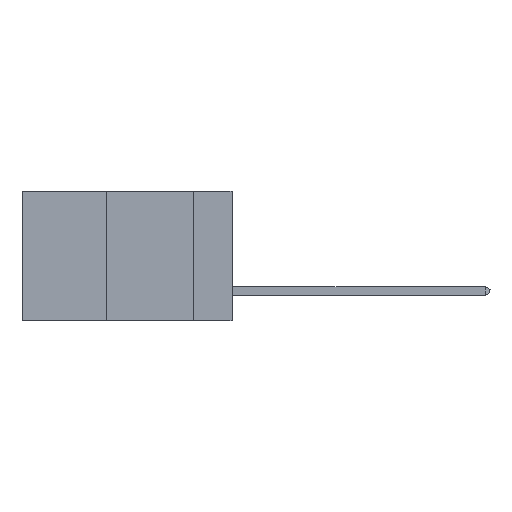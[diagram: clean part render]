
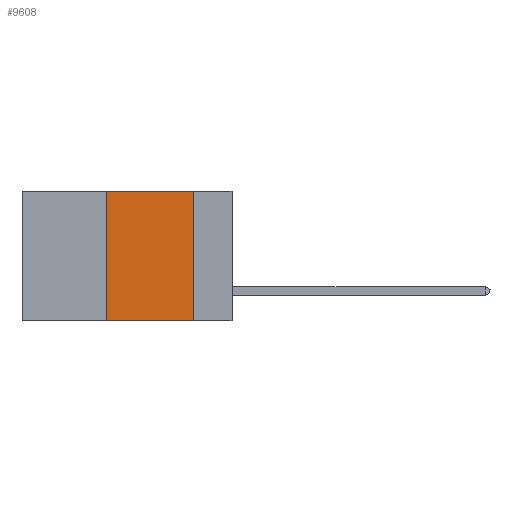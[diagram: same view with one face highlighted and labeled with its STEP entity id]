
A CAD part, left-side view. The second image highlights one B-rep face of the part: STEP entity #9608.
In plain terms, the highlighted planar face has unit normal (-1, 0, 0).
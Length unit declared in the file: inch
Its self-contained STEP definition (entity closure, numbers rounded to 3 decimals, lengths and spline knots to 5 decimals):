
#503 = DIRECTION ( 'NONE',  ( 0., -1., 0. ) ) ;
#2063 = CARTESIAN_POINT ( 'NONE',  ( 0., 0.11, 0. ) ) ;
#2697 = CARTESIAN_POINT ( 'NONE',  ( 0., 0.36, 0. ) ) ;
#3089 = EDGE_CURVE ( 'NONE', #4836, #41034, #37772, .T. ) ;
#3091 = DIRECTION ( 'NONE',  ( 0., -1., 0. ) ) ;
#3403 = CARTESIAN_POINT ( 'NONE',  ( 0., 0.6, 0. ) ) ;
#4161 = CARTESIAN_POINT ( 'NONE',  ( 0., 0.6, -0.37 ) ) ;
#4836 = VERTEX_POINT ( 'NONE', #2063 ) ;
#5991 = LINE ( 'NONE', #4161, #6514 ) ;
#6039 = CARTESIAN_POINT ( 'NONE',  ( 0., 0.6, 0. ) ) ;
#6367 = VECTOR ( 'NONE', #20189, 39.37008 ) ;
#6514 = VECTOR ( 'NONE', #503, 39.37008 ) ;
#7073 = EDGE_CURVE ( 'NONE', #39208, #4836, #10247, .T. ) ;
#7361 = ORIENTED_EDGE ( 'NONE', *, *, #29477, .T. ) ;
#8888 = VECTOR ( 'NONE', #37668, 39.37008 ) ;
#9069 = DIRECTION ( 'NONE',  ( 0., 0., -1. ) ) ;
#9608 = ADVANCED_FACE ( 'NONE', ( #11152 ), #29910, .F. ) ;
#10247 = LINE ( 'NONE', #3403, #39128 ) ;
#10647 = AXIS2_PLACEMENT_3D ( 'NONE', #6039, #33716, #9069 ) ;
#10871 = EDGE_CURVE ( 'NONE', #35455, #39208, #38512, .T. ) ;
#11152 = FACE_OUTER_BOUND ( 'NONE', #34648, .T. ) ;
#12516 = ORIENTED_EDGE ( 'NONE', *, *, #7073, .F. ) ;
#15843 = ORIENTED_EDGE ( 'NONE', *, *, #3089, .F. ) ;
#17462 = ORIENTED_EDGE ( 'NONE', *, *, #10871, .F. ) ;
#20189 = DIRECTION ( 'NONE',  ( 0., 0., 1. ) ) ;
#20245 = CARTESIAN_POINT ( 'NONE',  ( 0., 0.11, 0. ) ) ;
#21768 = CARTESIAN_POINT ( 'NONE',  ( 0., 0.11, -0.37 ) ) ;
#22938 = CARTESIAN_POINT ( 'NONE',  ( 0., 0.36, 0. ) ) ;
#23489 = CARTESIAN_POINT ( 'NONE',  ( 0., 0.36, -0.37 ) ) ;
#29477 = EDGE_CURVE ( 'NONE', #35455, #41034, #5991, .T. ) ;
#29910 = PLANE ( 'NONE',  #10647 ) ;
#33716 = DIRECTION ( 'NONE',  ( 1., 0., 0. ) ) ;
#34648 = EDGE_LOOP ( 'NONE', ( #15843, #12516, #17462, #7361 ) ) ;
#35455 = VERTEX_POINT ( 'NONE', #23489 ) ;
#37668 = DIRECTION ( 'NONE',  ( 0., 0., -1. ) ) ;
#37772 = LINE ( 'NONE', #20245, #8888 ) ;
#38512 = LINE ( 'NONE', #22938, #6367 ) ;
#39128 = VECTOR ( 'NONE', #3091, 39.37008 ) ;
#39208 = VERTEX_POINT ( 'NONE', #2697 ) ;
#41034 = VERTEX_POINT ( 'NONE', #21768 ) ;
